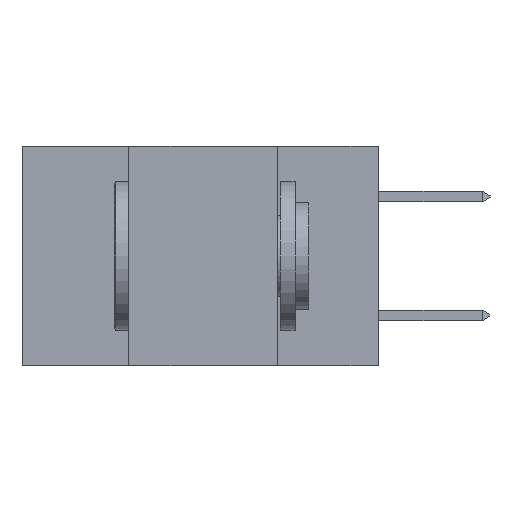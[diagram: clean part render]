
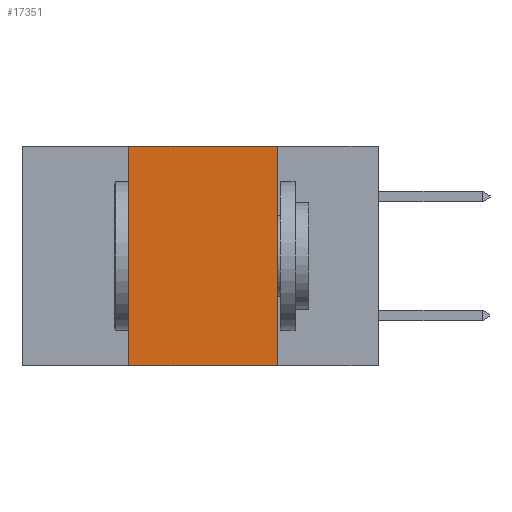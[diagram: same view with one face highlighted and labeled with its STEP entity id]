
A CAD part, left-side view. The second image highlights one B-rep face of the part: STEP entity #17351.
In plain terms, the highlighted planar face has unit normal (-1, 0, 0).
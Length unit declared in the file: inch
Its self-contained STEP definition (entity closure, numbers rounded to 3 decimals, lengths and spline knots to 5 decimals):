
#369 = CARTESIAN_POINT ( 'NONE',  ( 0., 0.17, 0. ) ) ;
#3451 = EDGE_CURVE ( 'NONE', #21000, #21855, #17770, .T. ) ;
#4792 = PLANE ( 'NONE',  #22349 ) ;
#5768 = VECTOR ( 'NONE', #21302, 39.37008 ) ;
#6761 = CARTESIAN_POINT ( 'NONE',  ( 0., 0.42, -0.37 ) ) ;
#7317 = CARTESIAN_POINT ( 'NONE',  ( 0., 0.17, -0.37 ) ) ;
#8132 = CARTESIAN_POINT ( 'NONE',  ( 0., 0.42, 0. ) ) ;
#8206 = CARTESIAN_POINT ( 'NONE',  ( 0., 0.6, -0.37 ) ) ;
#8460 = ORIENTED_EDGE ( 'NONE', *, *, #3451, .T. ) ;
#8760 = LINE ( 'NONE', #8132, #20412 ) ;
#8812 = ORIENTED_EDGE ( 'NONE', *, *, #15021, .F. ) ;
#9467 = DIRECTION ( 'NONE',  ( 0., 0., -1. ) ) ;
#9588 = CARTESIAN_POINT ( 'NONE',  ( 0., 0.42, 0. ) ) ;
#10445 = DIRECTION ( 'NONE',  ( 0., 0., 1. ) ) ;
#11264 = EDGE_CURVE ( 'NONE', #21000, #30121, #8760, .T. ) ;
#12229 = EDGE_CURVE ( 'NONE', #16616, #21855, #23658, .T. ) ;
#13905 = DIRECTION ( 'NONE',  ( 0., -1., 0. ) ) ;
#15021 = EDGE_CURVE ( 'NONE', #30121, #16616, #24498, .T. ) ;
#16209 = DIRECTION ( 'NONE',  ( 0., -1., 0. ) ) ;
#16616 = VERTEX_POINT ( 'NONE', #21105 ) ;
#17041 = VECTOR ( 'NONE', #16209, 39.37008 ) ;
#17351 = ADVANCED_FACE ( 'NONE', ( #29512 ), #4792, .F. ) ;
#17770 = LINE ( 'NONE', #8206, #17041 ) ;
#17812 = EDGE_LOOP ( 'NONE', ( #25245, #8812, #28166, #8460 ) ) ;
#20412 = VECTOR ( 'NONE', #10445, 39.37008 ) ;
#21000 = VERTEX_POINT ( 'NONE', #6761 ) ;
#21071 = CARTESIAN_POINT ( 'NONE',  ( 0., 0.6, 0. ) ) ;
#21105 = CARTESIAN_POINT ( 'NONE',  ( 0., 0.17, 0. ) ) ;
#21302 = DIRECTION ( 'NONE',  ( 0., 0., -1. ) ) ;
#21855 = VERTEX_POINT ( 'NONE', #7317 ) ;
#22349 = AXIS2_PLACEMENT_3D ( 'NONE', #21071, #23450, #9467 ) ;
#23450 = DIRECTION ( 'NONE',  ( 1., 0., 0. ) ) ;
#23658 = LINE ( 'NONE', #369, #5768 ) ;
#24498 = LINE ( 'NONE', #27962, #25221 ) ;
#25221 = VECTOR ( 'NONE', #13905, 39.37008 ) ;
#25245 = ORIENTED_EDGE ( 'NONE', *, *, #12229, .F. ) ;
#27962 = CARTESIAN_POINT ( 'NONE',  ( 0., 0.6, 0. ) ) ;
#28166 = ORIENTED_EDGE ( 'NONE', *, *, #11264, .F. ) ;
#29512 = FACE_OUTER_BOUND ( 'NONE', #17812, .T. ) ;
#30121 = VERTEX_POINT ( 'NONE', #9588 ) ;
